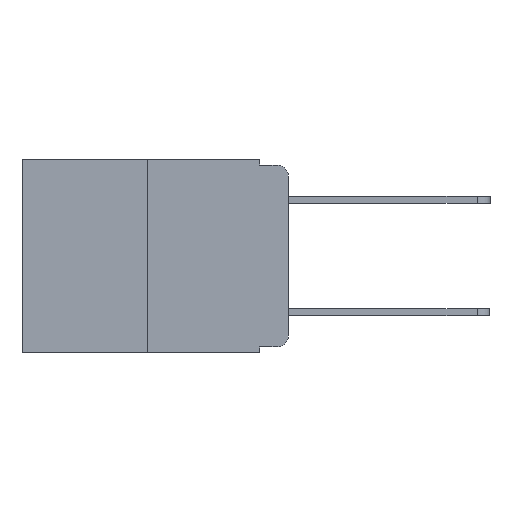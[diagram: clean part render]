
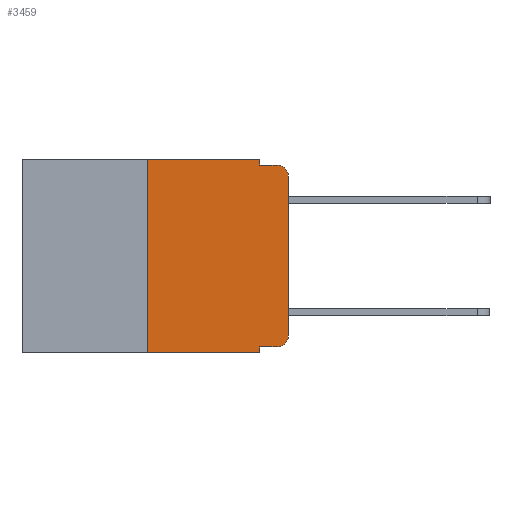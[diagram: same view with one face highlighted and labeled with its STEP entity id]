
A CAD part, left-side view. The second image highlights one B-rep face of the part: STEP entity #3459.
In plain terms, the highlighted planar face has unit normal (-1, 0, 0).
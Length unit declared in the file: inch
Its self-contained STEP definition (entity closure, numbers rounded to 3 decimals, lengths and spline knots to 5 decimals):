
#18 = FACE_OUTER_BOUND ( 'NONE', #12055, .T. ) ;
#385 = DIRECTION ( 'NONE',  ( 0., -1., 0. ) ) ;
#607 = CARTESIAN_POINT ( 'NONE',  ( 0., 0.25, -0.343 ) ) ;
#715 = CARTESIAN_POINT ( 'NONE',  ( 0., 0.051, -0.01 ) ) ;
#1004 = LINE ( 'NONE', #14094, #1476 ) ;
#1432 = VERTEX_POINT ( 'NONE', #1803 ) ;
#1476 = VECTOR ( 'NONE', #5401, 39.37008 ) ;
#1803 = CARTESIAN_POINT ( 'NONE',  ( 0., 0.02, -0.01 ) ) ;
#1966 = LINE ( 'NONE', #4304, #17058 ) ;
#2002 = VERTEX_POINT ( 'NONE', #2180 ) ;
#2129 = DIRECTION ( 'NONE',  ( 0., 0., -1. ) ) ;
#2180 = CARTESIAN_POINT ( 'NONE',  ( 0., 0., -0.03 ) ) ;
#2198 = DIRECTION ( 'NONE',  ( 0., -1., 0. ) ) ;
#2535 = VERTEX_POINT ( 'NONE', #6536 ) ;
#2567 = DIRECTION ( 'NONE',  ( 1., 0., 0. ) ) ;
#2703 = VECTOR ( 'NONE', #18289, 39.37008 ) ;
#2745 = AXIS2_PLACEMENT_3D ( 'NONE', #8327, #18551, #9775 ) ;
#2780 = PLANE ( 'NONE',  #13854 ) ;
#3045 = ORIENTED_EDGE ( 'NONE', *, *, #9943, .T. ) ;
#3080 = LINE ( 'NONE', #11952, #9908 ) ;
#3444 = ORIENTED_EDGE ( 'NONE', *, *, #17892, .T. ) ;
#3459 = ADVANCED_FACE ( 'NONE', ( #18 ), #2780, .F. ) ;
#3460 = VERTEX_POINT ( 'NONE', #16668 ) ;
#3731 = LINE ( 'NONE', #715, #14883 ) ;
#4304 = CARTESIAN_POINT ( 'NONE',  ( 0., 0.051, 0. ) ) ;
#4565 = CARTESIAN_POINT ( 'NONE',  ( 0., 0.02, -0.03 ) ) ;
#4603 = DIRECTION ( 'NONE',  ( 0., 0., -1. ) ) ;
#4777 = LINE ( 'NONE', #13074, #8621 ) ;
#5401 = DIRECTION ( 'NONE',  ( 0., -1., 0. ) ) ;
#5583 = EDGE_CURVE ( 'NONE', #2535, #2002, #4777, .T. ) ;
#5592 = AXIS2_PLACEMENT_3D ( 'NONE', #4565, #14731, #6013 ) ;
#5847 = VERTEX_POINT ( 'NONE', #16503 ) ;
#5981 = ORIENTED_EDGE ( 'NONE', *, *, #7692, .F. ) ;
#6005 = ORIENTED_EDGE ( 'NONE', *, *, #15807, .F. ) ;
#6013 = DIRECTION ( 'NONE',  ( 0., 0., -1. ) ) ;
#6016 = CARTESIAN_POINT ( 'NONE',  ( 0., 0.051, 0. ) ) ;
#6165 = DIRECTION ( 'NONE',  ( 0., 0., -1. ) ) ;
#6536 = CARTESIAN_POINT ( 'NONE',  ( 0., 0., -0.313 ) ) ;
#6594 = CARTESIAN_POINT ( 'NONE',  ( 0., 0.473, 0. ) ) ;
#7692 = EDGE_CURVE ( 'NONE', #13212, #3460, #3080, .T. ) ;
#7882 = LINE ( 'NONE', #13549, #15670 ) ;
#8155 = ORIENTED_EDGE ( 'NONE', *, *, #9069, .T. ) ;
#8241 = CARTESIAN_POINT ( 'NONE',  ( 0., 0.051, -0.333 ) ) ;
#8327 = CARTESIAN_POINT ( 'NONE',  ( 0., 0.02, -0.313 ) ) ;
#8621 = VECTOR ( 'NONE', #15948, 39.37008 ) ;
#9069 = EDGE_CURVE ( 'NONE', #11339, #2535, #15088, .T. ) ;
#9775 = DIRECTION ( 'NONE',  ( 0., 0., -1. ) ) ;
#9908 = VECTOR ( 'NONE', #6165, 39.37008 ) ;
#9943 = EDGE_CURVE ( 'NONE', #2002, #1432, #16423, .T. ) ;
#10750 = EDGE_CURVE ( 'NONE', #17560, #13212, #18230, .T. ) ;
#11100 = CARTESIAN_POINT ( 'NONE',  ( 0., 0.25, 0. ) ) ;
#11339 = VERTEX_POINT ( 'NONE', #16138 ) ;
#11585 = ORIENTED_EDGE ( 'NONE', *, *, #17760, .F. ) ;
#11855 = VECTOR ( 'NONE', #18643, 39.37008 ) ;
#11952 = CARTESIAN_POINT ( 'NONE',  ( 0., 0.051, 0. ) ) ;
#12055 = EDGE_LOOP ( 'NONE', ( #13859, #3045, #15521, #5981, #16803, #6005, #17784, #11585, #3444, #8155 ) ) ;
#12756 = CARTESIAN_POINT ( 'NONE',  ( 0., 0.25, 0. ) ) ;
#13074 = CARTESIAN_POINT ( 'NONE',  ( 0., 0., 0. ) ) ;
#13212 = VERTEX_POINT ( 'NONE', #6016 ) ;
#13549 = CARTESIAN_POINT ( 'NONE',  ( 0., 0.051, -0.333 ) ) ;
#13854 = AXIS2_PLACEMENT_3D ( 'NONE', #16809, #2567, #2129 ) ;
#13859 = ORIENTED_EDGE ( 'NONE', *, *, #5583, .T. ) ;
#14094 = CARTESIAN_POINT ( 'NONE',  ( 0., 0.473, -0.343 ) ) ;
#14731 = DIRECTION ( 'NONE',  ( -1., 0., 0. ) ) ;
#14883 = VECTOR ( 'NONE', #2198, 39.37008 ) ;
#14985 = EDGE_CURVE ( 'NONE', #3460, #1432, #3731, .T. ) ;
#15088 = CIRCLE ( 'NONE', #2745, 0.02 ) ;
#15521 = ORIENTED_EDGE ( 'NONE', *, *, #14985, .F. ) ;
#15670 = VECTOR ( 'NONE', #385, 39.37008 ) ;
#15716 = VERTEX_POINT ( 'NONE', #8241 ) ;
#15765 = LINE ( 'NONE', #12756, #11855 ) ;
#15807 = EDGE_CURVE ( 'NONE', #16149, #17560, #15765, .T. ) ;
#15948 = DIRECTION ( 'NONE',  ( 0., 0., 1. ) ) ;
#16138 = CARTESIAN_POINT ( 'NONE',  ( 0., 0.02, -0.333 ) ) ;
#16149 = VERTEX_POINT ( 'NONE', #607 ) ;
#16423 = CIRCLE ( 'NONE', #5592, 0.02 ) ;
#16503 = CARTESIAN_POINT ( 'NONE',  ( 0., 0.051, -0.343 ) ) ;
#16668 = CARTESIAN_POINT ( 'NONE',  ( 0., 0.051, -0.01 ) ) ;
#16803 = ORIENTED_EDGE ( 'NONE', *, *, #10750, .F. ) ;
#16809 = CARTESIAN_POINT ( 'NONE',  ( 0., 0.473, 0. ) ) ;
#17058 = VECTOR ( 'NONE', #4603, 39.37008 ) ;
#17560 = VERTEX_POINT ( 'NONE', #11100 ) ;
#17760 = EDGE_CURVE ( 'NONE', #15716, #5847, #1966, .T. ) ;
#17784 = ORIENTED_EDGE ( 'NONE', *, *, #18720, .T. ) ;
#17892 = EDGE_CURVE ( 'NONE', #15716, #11339, #7882, .T. ) ;
#18230 = LINE ( 'NONE', #6594, #2703 ) ;
#18289 = DIRECTION ( 'NONE',  ( 0., -1., 0. ) ) ;
#18551 = DIRECTION ( 'NONE',  ( -1., 0., 0. ) ) ;
#18643 = DIRECTION ( 'NONE',  ( 0., 0., 1. ) ) ;
#18720 = EDGE_CURVE ( 'NONE', #16149, #5847, #1004, .T. ) ;
